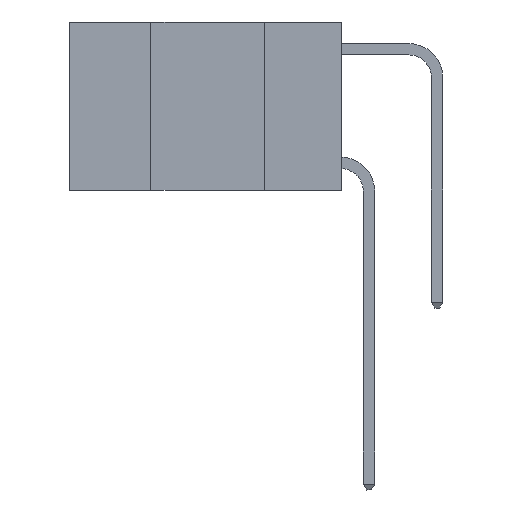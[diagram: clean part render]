
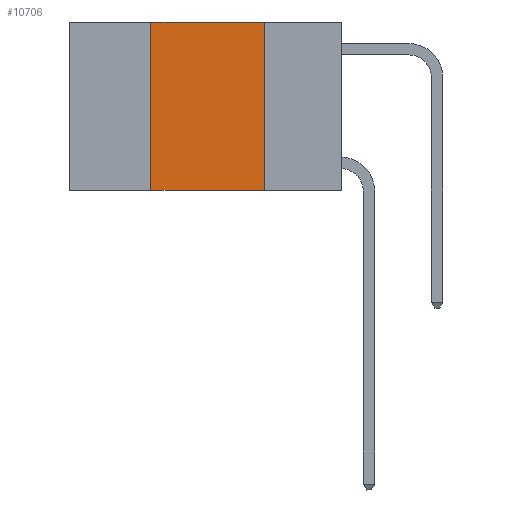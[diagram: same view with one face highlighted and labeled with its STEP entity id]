
A CAD part, left-side view. The second image highlights one B-rep face of the part: STEP entity #10706.
In plain terms, the highlighted planar face has unit normal (-1, 0, 0).
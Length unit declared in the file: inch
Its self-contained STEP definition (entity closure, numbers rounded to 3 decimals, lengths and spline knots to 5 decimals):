
#302 = CARTESIAN_POINT ( 'NONE',  ( 0., 0.17, 0. ) ) ;
#972 = EDGE_CURVE ( 'NONE', #14272, #6738, #11732, .T. ) ;
#2244 = VECTOR ( 'NONE', #9182, 39.37008 ) ;
#2557 = DIRECTION ( 'NONE',  ( 0., -1., 0. ) ) ;
#3053 = LINE ( 'NONE', #10993, #5901 ) ;
#3087 = CARTESIAN_POINT ( 'NONE',  ( 0., 0.6, 0. ) ) ;
#3230 = FACE_OUTER_BOUND ( 'NONE', #7463, .T. ) ;
#3455 = VERTEX_POINT ( 'NONE', #11906 ) ;
#4275 = DIRECTION ( 'NONE',  ( 0., 0., -1. ) ) ;
#4546 = ORIENTED_EDGE ( 'NONE', *, *, #13901, .F. ) ;
#4786 = LINE ( 'NONE', #12887, #9511 ) ;
#5109 = CARTESIAN_POINT ( 'NONE',  ( 0., 0.6, -0.37 ) ) ;
#5171 = EDGE_CURVE ( 'NONE', #14272, #14138, #3053, .T. ) ;
#5850 = CARTESIAN_POINT ( 'NONE',  ( 0., 0.42, -0.37 ) ) ;
#5901 = VECTOR ( 'NONE', #10914, 39.37008 ) ;
#5977 = DIRECTION ( 'NONE',  ( 0., -1., 0. ) ) ;
#6604 = CARTESIAN_POINT ( 'NONE',  ( 0., 0.42, 0. ) ) ;
#6620 = DIRECTION ( 'NONE',  ( 1., 0., 0. ) ) ;
#6738 = VERTEX_POINT ( 'NONE', #13781 ) ;
#7463 = EDGE_LOOP ( 'NONE', ( #12792, #4546, #14006, #12592 ) ) ;
#7737 = PLANE ( 'NONE',  #11621 ) ;
#9182 = DIRECTION ( 'NONE',  ( 0., 0., -1. ) ) ;
#9511 = VECTOR ( 'NONE', #2557, 39.37008 ) ;
#9795 = EDGE_CURVE ( 'NONE', #3455, #6738, #12503, .T. ) ;
#10706 = ADVANCED_FACE ( 'NONE', ( #3230 ), #7737, .F. ) ;
#10914 = DIRECTION ( 'NONE',  ( 0., 0., 1. ) ) ;
#10993 = CARTESIAN_POINT ( 'NONE',  ( 0., 0.42, 0. ) ) ;
#11621 = AXIS2_PLACEMENT_3D ( 'NONE', #3087, #6620, #4275 ) ;
#11732 = LINE ( 'NONE', #5109, #13204 ) ;
#11906 = CARTESIAN_POINT ( 'NONE',  ( 0., 0.17, 0. ) ) ;
#12503 = LINE ( 'NONE', #302, #2244 ) ;
#12592 = ORIENTED_EDGE ( 'NONE', *, *, #972, .T. ) ;
#12792 = ORIENTED_EDGE ( 'NONE', *, *, #9795, .F. ) ;
#12887 = CARTESIAN_POINT ( 'NONE',  ( 0., 0.6, 0. ) ) ;
#13204 = VECTOR ( 'NONE', #5977, 39.37008 ) ;
#13781 = CARTESIAN_POINT ( 'NONE',  ( 0., 0.17, -0.37 ) ) ;
#13901 = EDGE_CURVE ( 'NONE', #14138, #3455, #4786, .T. ) ;
#14006 = ORIENTED_EDGE ( 'NONE', *, *, #5171, .F. ) ;
#14138 = VERTEX_POINT ( 'NONE', #6604 ) ;
#14272 = VERTEX_POINT ( 'NONE', #5850 ) ;
